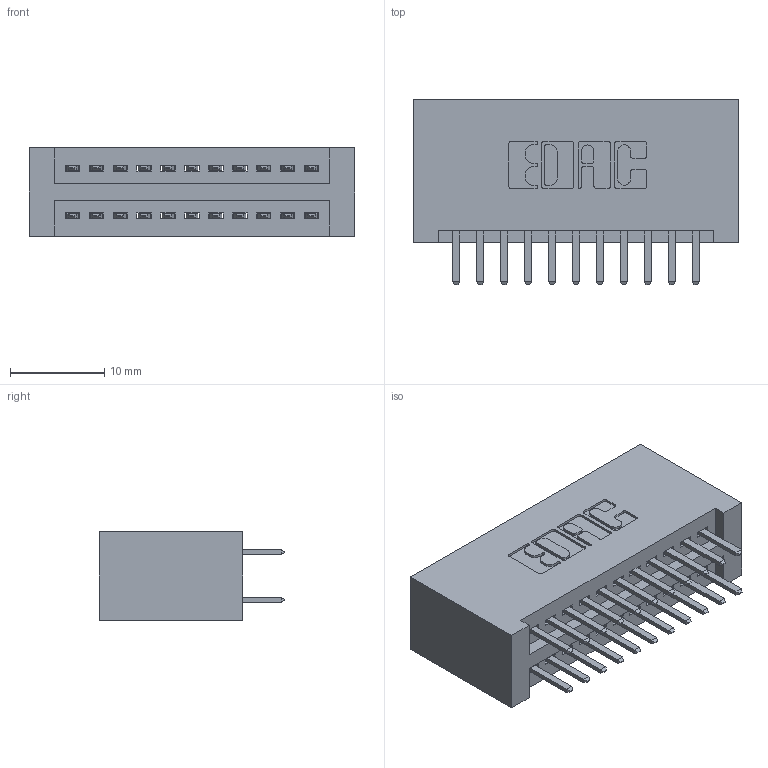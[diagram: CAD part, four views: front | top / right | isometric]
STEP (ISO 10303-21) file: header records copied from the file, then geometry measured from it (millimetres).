
FILE_DESCRIPTION (( 'STEP AP203' ), '1' );
FILE_NAME ('345-022-520-201.STEP', '2018-08-20T11:01:02', ( '' ), ( '' ), 'SwSTEP 2.0', 'SolidWorks 2016', '' );
FILE_SCHEMA (( 'CONFIG_CONTROL_DESIGN' ));
Length unit declared in the file: inch
Products named in the file (3): 345 Part_No Mounting Lugs; 345-292-001_345-293-120; 345-022-520-201
Assembly tree (23 placements, depth 2):
  345-022-520-201
    345 Part_No Mounting Lugs
    345-292-001_345-293-120  x22
Bounding box: 34.54 x 19.68 x 9.4 mm (x, y, z)
Volume: 3674.1 mm3; surface area: 5113.3 mm2
Topology: 23 solids, 23 shells, 1306 faces, 3771 edges, 2454 vertices
Faces by surface type: plane 846, cylinder 460
Entity records: 12641 total; most frequent: CARTESIAN_POINT 2160, ORIENTED_EDGE 2082, DIRECTION 1925, EDGE_CURVE 1041, LINE 869, VECTOR 869, VERTEX_POINT 690, AXIS2_PLACEMENT_3D 528
